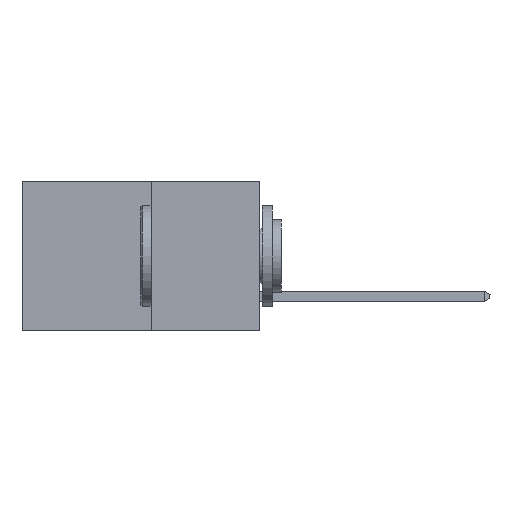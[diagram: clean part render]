
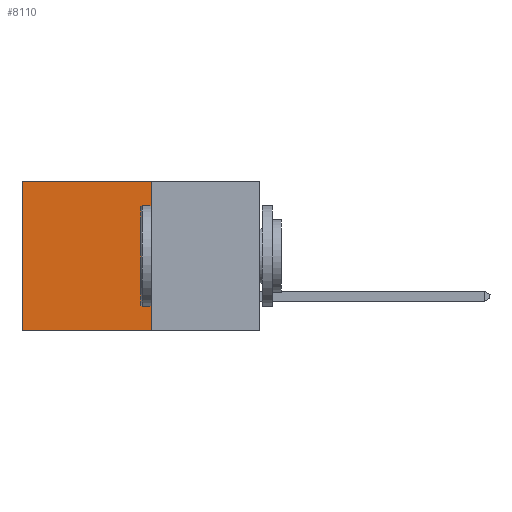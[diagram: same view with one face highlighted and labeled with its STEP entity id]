
A CAD part, left-side view. The second image highlights one B-rep face of the part: STEP entity #8110.
In plain terms, the highlighted planar face has unit normal (-1, 0, 0).
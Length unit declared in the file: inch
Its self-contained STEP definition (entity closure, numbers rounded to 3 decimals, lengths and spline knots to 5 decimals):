
#99 = DIRECTION ( 'NONE',  ( 1., 0., 0. ) ) ;
#402 = CARTESIAN_POINT ( 'NONE',  ( 0.277, 0.59, 0. ) ) ;
#1905 = ORIENTED_EDGE ( 'NONE', *, *, #5396, .T. ) ;
#1986 = VECTOR ( 'NONE', #2171, 39.37008 ) ;
#1998 = VERTEX_POINT ( 'NONE', #402 ) ;
#2079 = VECTOR ( 'NONE', #9021, 39.37008 ) ;
#2171 = DIRECTION ( 'NONE',  ( 0., 1., 0. ) ) ;
#2240 = CARTESIAN_POINT ( 'NONE',  ( 0.277, 0.59, -0.37 ) ) ;
#2394 = LINE ( 'NONE', #9138, #2079 ) ;
#2480 = EDGE_CURVE ( 'NONE', #4396, #6163, #2394, .T. ) ;
#2583 = DIRECTION ( 'NONE',  ( 0., 1., 0. ) ) ;
#2679 = EDGE_CURVE ( 'NONE', #4396, #1998, #11228, .T. ) ;
#2705 = AXIS2_PLACEMENT_3D ( 'NONE', #5903, #99, #6830 ) ;
#2886 = CARTESIAN_POINT ( 'NONE',  ( 0.277, 0.27, 0. ) ) ;
#2905 = LINE ( 'NONE', #10047, #5135 ) ;
#4396 = VERTEX_POINT ( 'NONE', #5284 ) ;
#4483 = LINE ( 'NONE', #5878, #1986 ) ;
#4800 = CARTESIAN_POINT ( 'NONE',  ( 0.277, 0.27, -0.37 ) ) ;
#5055 = FACE_OUTER_BOUND ( 'NONE', #9897, .T. ) ;
#5135 = VECTOR ( 'NONE', #9947, 39.37008 ) ;
#5284 = CARTESIAN_POINT ( 'NONE',  ( 0.277, 0.27, 0. ) ) ;
#5396 = EDGE_CURVE ( 'NONE', #1998, #6452, #2905, .T. ) ;
#5845 = ORIENTED_EDGE ( 'NONE', *, *, #2480, .F. ) ;
#5878 = CARTESIAN_POINT ( 'NONE',  ( 0.277, 0.27, -0.37 ) ) ;
#5903 = CARTESIAN_POINT ( 'NONE',  ( 0.277, 0.27, -0.37 ) ) ;
#6163 = VERTEX_POINT ( 'NONE', #4800 ) ;
#6452 = VERTEX_POINT ( 'NONE', #2240 ) ;
#6830 = DIRECTION ( 'NONE',  ( 0., 0., -1. ) ) ;
#7290 = EDGE_CURVE ( 'NONE', #6163, #6452, #4483, .T. ) ;
#8110 = ADVANCED_FACE ( 'NONE', ( #5055 ), #10052, .F. ) ;
#9021 = DIRECTION ( 'NONE',  ( 0., 0., -1. ) ) ;
#9031 = VECTOR ( 'NONE', #2583, 39.37008 ) ;
#9138 = CARTESIAN_POINT ( 'NONE',  ( 0.277, 0.27, -0.37 ) ) ;
#9897 = EDGE_LOOP ( 'NONE', ( #1905, #11459, #5845, #11587 ) ) ;
#9947 = DIRECTION ( 'NONE',  ( 0., 0., -1. ) ) ;
#10047 = CARTESIAN_POINT ( 'NONE',  ( 0.277, 0.59, -0.37 ) ) ;
#10052 = PLANE ( 'NONE',  #2705 ) ;
#11228 = LINE ( 'NONE', #2886, #9031 ) ;
#11459 = ORIENTED_EDGE ( 'NONE', *, *, #7290, .F. ) ;
#11587 = ORIENTED_EDGE ( 'NONE', *, *, #2679, .T. ) ;
